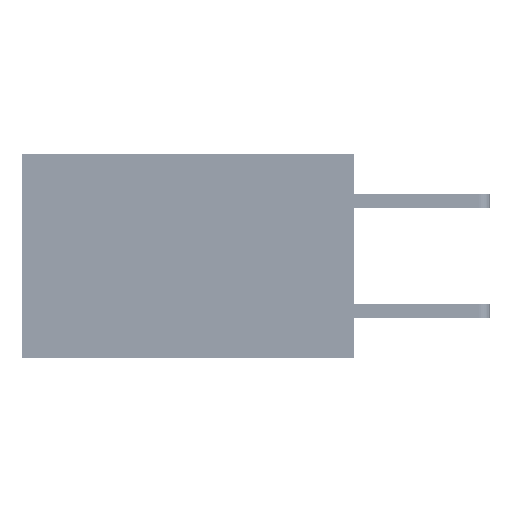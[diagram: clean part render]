
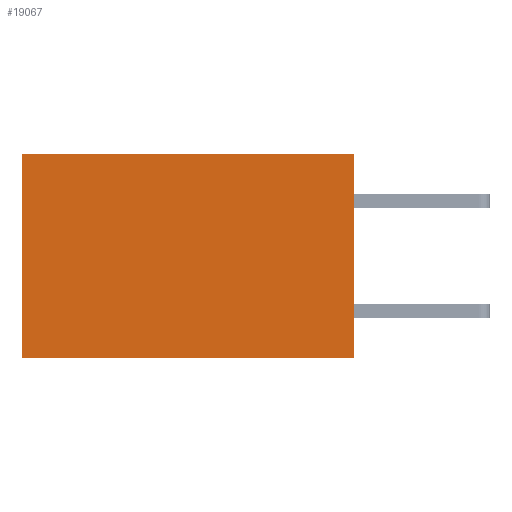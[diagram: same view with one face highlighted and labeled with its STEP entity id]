
A CAD part, left-side view. The second image highlights one B-rep face of the part: STEP entity #19067.
In plain terms, the highlighted planar face has unit normal (-1, 0, 0).
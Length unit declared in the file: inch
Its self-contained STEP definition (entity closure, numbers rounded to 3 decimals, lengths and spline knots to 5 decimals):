
#958 = VECTOR ( 'NONE', #33615, 39.37008 ) ;
#2253 = DIRECTION ( 'NONE',  ( 1., 0., 0. ) ) ;
#2577 = VECTOR ( 'NONE', #29979, 39.37008 ) ;
#4032 = CARTESIAN_POINT ( 'NONE',  ( 0.2875, 0., 0. ) ) ;
#4430 = CARTESIAN_POINT ( 'NONE',  ( 0.2875, 0., 0. ) ) ;
#5129 = LINE ( 'NONE', #10747, #958 ) ;
#5241 = DIRECTION ( 'NONE',  ( 0., 1., 0. ) ) ;
#5611 = PLANE ( 'NONE',  #32321 ) ;
#7334 = CARTESIAN_POINT ( 'NONE',  ( 0.2875, 0., -0.37 ) ) ;
#7555 = EDGE_CURVE ( 'NONE', #11758, #24289, #37858, .T. ) ;
#8445 = EDGE_CURVE ( 'NONE', #15875, #36093, #5129, .T. ) ;
#10747 = CARTESIAN_POINT ( 'NONE',  ( 0.2875, 0., 0. ) ) ;
#11758 = VERTEX_POINT ( 'NONE', #40882 ) ;
#12898 = CARTESIAN_POINT ( 'NONE',  ( 0.2875, 0.6, -0.37 ) ) ;
#13585 = EDGE_CURVE ( 'NONE', #15875, #11758, #38086, .T. ) ;
#15875 = VERTEX_POINT ( 'NONE', #4032 ) ;
#17350 = CARTESIAN_POINT ( 'NONE',  ( 0.2875, 0., 0. ) ) ;
#19067 = ADVANCED_FACE ( 'NONE', ( #39814 ), #5611, .F. ) ;
#22107 = CARTESIAN_POINT ( 'NONE',  ( 0.2875, 0., -0.37 ) ) ;
#23024 = VECTOR ( 'NONE', #5241, 39.37008 ) ;
#24161 = VECTOR ( 'NONE', #30703, 39.37008 ) ;
#24289 = VERTEX_POINT ( 'NONE', #12898 ) ;
#25577 = ORIENTED_EDGE ( 'NONE', *, *, #8445, .F. ) ;
#26111 = CARTESIAN_POINT ( 'NONE',  ( 0.2875, 0.6, 0. ) ) ;
#26602 = ORIENTED_EDGE ( 'NONE', *, *, #7555, .T. ) ;
#29979 = DIRECTION ( 'NONE',  ( 0., 0., -1. ) ) ;
#30703 = DIRECTION ( 'NONE',  ( 0., 1., 0. ) ) ;
#32316 = LINE ( 'NONE', #22107, #23024 ) ;
#32321 = AXIS2_PLACEMENT_3D ( 'NONE', #4430, #2253, #38378 ) ;
#32322 = ORIENTED_EDGE ( 'NONE', *, *, #13585, .T. ) ;
#32682 = ORIENTED_EDGE ( 'NONE', *, *, #36554, .F. ) ;
#33511 = EDGE_LOOP ( 'NONE', ( #26602, #32682, #25577, #32322 ) ) ;
#33615 = DIRECTION ( 'NONE',  ( 0., 0., -1. ) ) ;
#36093 = VERTEX_POINT ( 'NONE', #7334 ) ;
#36554 = EDGE_CURVE ( 'NONE', #36093, #24289, #32316, .T. ) ;
#37858 = LINE ( 'NONE', #26111, #2577 ) ;
#38086 = LINE ( 'NONE', #17350, #24161 ) ;
#38378 = DIRECTION ( 'NONE',  ( 0., 0., -1. ) ) ;
#39814 = FACE_OUTER_BOUND ( 'NONE', #33511, .T. ) ;
#40882 = CARTESIAN_POINT ( 'NONE',  ( 0.2875, 0.6, 0. ) ) ;
